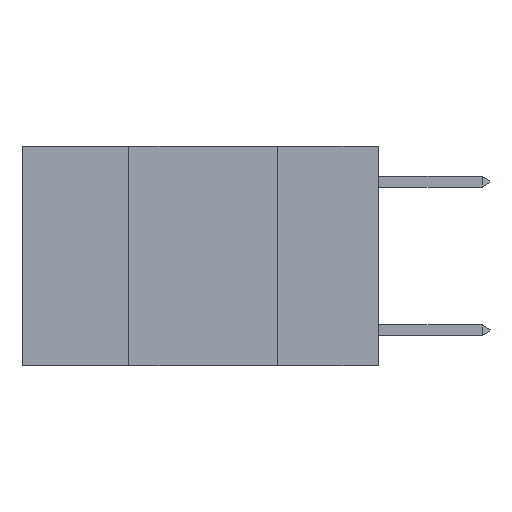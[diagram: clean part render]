
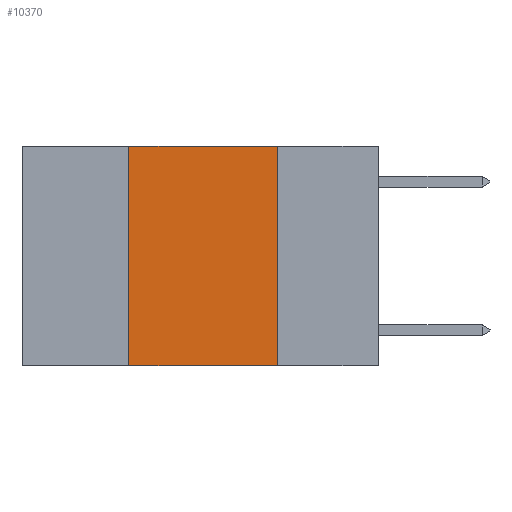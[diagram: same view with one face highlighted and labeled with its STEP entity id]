
A CAD part, left-side view. The second image highlights one B-rep face of the part: STEP entity #10370.
In plain terms, the highlighted planar face has unit normal (-1, 0, 0).
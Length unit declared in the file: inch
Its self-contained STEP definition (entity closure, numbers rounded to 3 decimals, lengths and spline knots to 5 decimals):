
#204 = LINE ( 'NONE', #14563, #11215 ) ;
#496 = ORIENTED_EDGE ( 'NONE', *, *, #24435, .F. ) ;
#539 = VECTOR ( 'NONE', #15682, 39.37008 ) ;
#2308 = FACE_OUTER_BOUND ( 'NONE', #17605, .T. ) ;
#4448 = LINE ( 'NONE', #9650, #25799 ) ;
#5752 = CARTESIAN_POINT ( 'NONE',  ( 0., 0.17, 0. ) ) ;
#6216 = ORIENTED_EDGE ( 'NONE', *, *, #25998, .F. ) ;
#7106 = VERTEX_POINT ( 'NONE', #20416 ) ;
#8687 = CARTESIAN_POINT ( 'NONE',  ( 0., 0.42, 0. ) ) ;
#9134 = VERTEX_POINT ( 'NONE', #10624 ) ;
#9650 = CARTESIAN_POINT ( 'NONE',  ( 0., 0.17, 0. ) ) ;
#10081 = PLANE ( 'NONE',  #22607 ) ;
#10370 = ADVANCED_FACE ( 'NONE', ( #2308 ), #10081, .F. ) ;
#10624 = CARTESIAN_POINT ( 'NONE',  ( 0., 0.42, -0.37 ) ) ;
#10836 = DIRECTION ( 'NONE',  ( 0., 0., 1. ) ) ;
#11215 = VECTOR ( 'NONE', #27063, 39.37008 ) ;
#12244 = DIRECTION ( 'NONE',  ( 1., 0., 0. ) ) ;
#13508 = ORIENTED_EDGE ( 'NONE', *, *, #21531, .T. ) ;
#13893 = CARTESIAN_POINT ( 'NONE',  ( 0., 0.17, -0.37 ) ) ;
#13897 = DIRECTION ( 'NONE',  ( 0., 0., -1. ) ) ;
#14563 = CARTESIAN_POINT ( 'NONE',  ( 0., 0.6, -0.37 ) ) ;
#15682 = DIRECTION ( 'NONE',  ( 0., -1., 0. ) ) ;
#17605 = EDGE_LOOP ( 'NONE', ( #496, #21913, #6216, #13508 ) ) ;
#17811 = CARTESIAN_POINT ( 'NONE',  ( 0., 0.6, 0. ) ) ;
#17891 = LINE ( 'NONE', #17811, #539 ) ;
#20040 = VERTEX_POINT ( 'NONE', #13893 ) ;
#20416 = CARTESIAN_POINT ( 'NONE',  ( 0., 0.42, 0. ) ) ;
#21531 = EDGE_CURVE ( 'NONE', #9134, #20040, #204, .T. ) ;
#21913 = ORIENTED_EDGE ( 'NONE', *, *, #25514, .F. ) ;
#22124 = VECTOR ( 'NONE', #10836, 39.37008 ) ;
#22487 = VERTEX_POINT ( 'NONE', #5752 ) ;
#22607 = AXIS2_PLACEMENT_3D ( 'NONE', #24903, #12244, #26929 ) ;
#22785 = LINE ( 'NONE', #8687, #22124 ) ;
#24435 = EDGE_CURVE ( 'NONE', #22487, #20040, #4448, .T. ) ;
#24903 = CARTESIAN_POINT ( 'NONE',  ( 0., 0.6, 0. ) ) ;
#25514 = EDGE_CURVE ( 'NONE', #7106, #22487, #17891, .T. ) ;
#25799 = VECTOR ( 'NONE', #13897, 39.37008 ) ;
#25998 = EDGE_CURVE ( 'NONE', #9134, #7106, #22785, .T. ) ;
#26929 = DIRECTION ( 'NONE',  ( 0., 0., -1. ) ) ;
#27063 = DIRECTION ( 'NONE',  ( 0., -1., 0. ) ) ;
